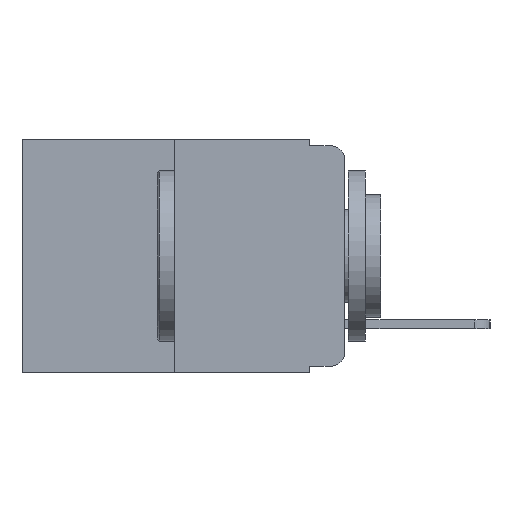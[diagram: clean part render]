
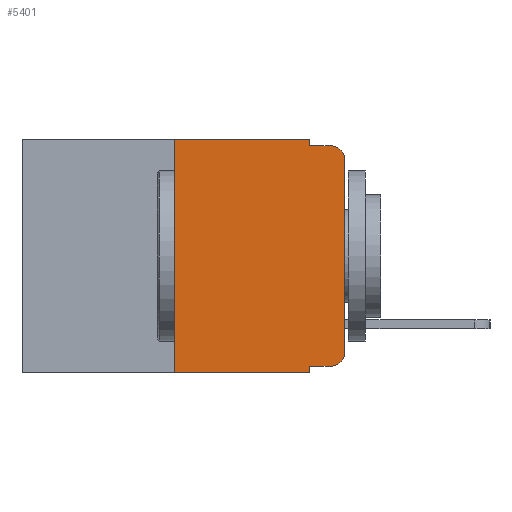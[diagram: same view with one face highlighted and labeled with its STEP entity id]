
A CAD part, left-side view. The second image highlights one B-rep face of the part: STEP entity #5401.
In plain terms, the highlighted planar face has unit normal (-1, 0, 0).
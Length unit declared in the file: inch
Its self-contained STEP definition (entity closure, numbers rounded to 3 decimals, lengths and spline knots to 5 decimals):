
#110 = VERTEX_POINT ( 'NONE', #2199 ) ;
#299 = DIRECTION ( 'NONE',  ( 0., 0., 1. ) ) ;
#365 = CARTESIAN_POINT ( 'NONE',  ( 0., 0.02, -0.01 ) ) ;
#613 = EDGE_CURVE ( 'NONE', #12020, #21949, #14878, .T. ) ;
#1210 = AXIS2_PLACEMENT_3D ( 'NONE', #22900, #11260, #24784 ) ;
#1240 = AXIS2_PLACEMENT_3D ( 'NONE', #11930, #15822, #15746 ) ;
#1742 = CARTESIAN_POINT ( 'NONE',  ( 0., 0.051, -0.01 ) ) ;
#2199 = CARTESIAN_POINT ( 'NONE',  ( 0., 0., -0.03 ) ) ;
#2797 = CARTESIAN_POINT ( 'NONE',  ( 0., 0.051, -0.333 ) ) ;
#2914 = VECTOR ( 'NONE', #299, 39.37008 ) ;
#2968 = DIRECTION ( 'NONE',  ( 0., 0., -1. ) ) ;
#3249 = VECTOR ( 'NONE', #24885, 39.37008 ) ;
#3741 = ORIENTED_EDGE ( 'NONE', *, *, #14303, .F. ) ;
#3817 = ORIENTED_EDGE ( 'NONE', *, *, #24107, .T. ) ;
#4139 = VECTOR ( 'NONE', #13583, 39.37008 ) ;
#5282 = CARTESIAN_POINT ( 'NONE',  ( 0., 0.051, -0.343 ) ) ;
#5379 = VECTOR ( 'NONE', #2968, 39.37008 ) ;
#5401 = ADVANCED_FACE ( 'NONE', ( #16788 ), #16209, .F. ) ;
#5691 = EDGE_CURVE ( 'NONE', #10953, #9320, #20780, .T. ) ;
#5709 = CARTESIAN_POINT ( 'NONE',  ( 0., 0.02, -0.313 ) ) ;
#6257 = CARTESIAN_POINT ( 'NONE',  ( 0., 0.051, 0. ) ) ;
#6479 = VERTEX_POINT ( 'NONE', #365 ) ;
#6507 = VERTEX_POINT ( 'NONE', #17838 ) ;
#7349 = VERTEX_POINT ( 'NONE', #8940 ) ;
#7655 = DIRECTION ( 'NONE',  ( 0., 0., -1. ) ) ;
#8054 = CARTESIAN_POINT ( 'NONE',  ( 0., 0., 0. ) ) ;
#8216 = LINE ( 'NONE', #22053, #17794 ) ;
#8354 = LINE ( 'NONE', #1742, #3249 ) ;
#8837 = CARTESIAN_POINT ( 'NONE',  ( 0., 0.051, -0.333 ) ) ;
#8940 = CARTESIAN_POINT ( 'NONE',  ( 0., 0.25, -0.343 ) ) ;
#8973 = EDGE_CURVE ( 'NONE', #10953, #19774, #20629, .T. ) ;
#9078 = VERTEX_POINT ( 'NONE', #19848 ) ;
#9320 = VERTEX_POINT ( 'NONE', #5282 ) ;
#10343 = VECTOR ( 'NONE', #18164, 39.37008 ) ;
#10953 = VERTEX_POINT ( 'NONE', #8837 ) ;
#11128 = ORIENTED_EDGE ( 'NONE', *, *, #24139, .T. ) ;
#11260 = DIRECTION ( 'NONE',  ( -1., 0., 0. ) ) ;
#11719 = CARTESIAN_POINT ( 'NONE',  ( 0., 0.473, -0.343 ) ) ;
#11804 = EDGE_CURVE ( 'NONE', #9078, #6479, #8354, .T. ) ;
#11930 = CARTESIAN_POINT ( 'NONE',  ( 0., 0.473, 0. ) ) ;
#12020 = VERTEX_POINT ( 'NONE', #16234 ) ;
#12696 = EDGE_CURVE ( 'NONE', #110, #6479, #20682, .T. ) ;
#12757 = CIRCLE ( 'NONE', #14114, 0.02 ) ;
#13583 = DIRECTION ( 'NONE',  ( 0., -1., 0. ) ) ;
#13606 = VECTOR ( 'NONE', #16019, 39.37008 ) ;
#14099 = CARTESIAN_POINT ( 'NONE',  ( 0., 0.25, 0. ) ) ;
#14114 = AXIS2_PLACEMENT_3D ( 'NONE', #5709, #19171, #7655 ) ;
#14237 = LINE ( 'NONE', #11719, #4139 ) ;
#14303 = EDGE_CURVE ( 'NONE', #21949, #9078, #8216, .T. ) ;
#14865 = ORIENTED_EDGE ( 'NONE', *, *, #8973, .T. ) ;
#14878 = LINE ( 'NONE', #24428, #24662 ) ;
#15746 = DIRECTION ( 'NONE',  ( 0., 0., -1. ) ) ;
#15822 = DIRECTION ( 'NONE',  ( 1., 0., 0. ) ) ;
#16019 = DIRECTION ( 'NONE',  ( 0., 0., 1. ) ) ;
#16209 = PLANE ( 'NONE',  #1240 ) ;
#16234 = CARTESIAN_POINT ( 'NONE',  ( 0., 0.25, 0. ) ) ;
#16788 = FACE_OUTER_BOUND ( 'NONE', #18303, .T. ) ;
#17525 = ORIENTED_EDGE ( 'NONE', *, *, #613, .F. ) ;
#17794 = VECTOR ( 'NONE', #23969, 39.37008 ) ;
#17838 = CARTESIAN_POINT ( 'NONE',  ( 0., 0., -0.313 ) ) ;
#18164 = DIRECTION ( 'NONE',  ( 0., -1., 0. ) ) ;
#18247 = ORIENTED_EDGE ( 'NONE', *, *, #5691, .F. ) ;
#18300 = ORIENTED_EDGE ( 'NONE', *, *, #23982, .T. ) ;
#18303 = EDGE_LOOP ( 'NONE', ( #11128, #20539, #22431, #3741, #17525, #22521, #3817, #18247, #14865, #18300 ) ) ;
#18834 = LINE ( 'NONE', #14099, #13606 ) ;
#18868 = LINE ( 'NONE', #8054, #2914 ) ;
#19171 = DIRECTION ( 'NONE',  ( -1., 0., 0. ) ) ;
#19272 = EDGE_CURVE ( 'NONE', #7349, #12020, #18834, .T. ) ;
#19774 = VERTEX_POINT ( 'NONE', #23449 ) ;
#19848 = CARTESIAN_POINT ( 'NONE',  ( 0., 0.051, -0.01 ) ) ;
#20539 = ORIENTED_EDGE ( 'NONE', *, *, #12696, .T. ) ;
#20629 = LINE ( 'NONE', #2797, #10343 ) ;
#20682 = CIRCLE ( 'NONE', #1210, 0.02 ) ;
#20780 = LINE ( 'NONE', #6257, #5379 ) ;
#21949 = VERTEX_POINT ( 'NONE', #24093 ) ;
#22053 = CARTESIAN_POINT ( 'NONE',  ( 0., 0.051, 0. ) ) ;
#22431 = ORIENTED_EDGE ( 'NONE', *, *, #11804, .F. ) ;
#22521 = ORIENTED_EDGE ( 'NONE', *, *, #19272, .F. ) ;
#22900 = CARTESIAN_POINT ( 'NONE',  ( 0., 0.02, -0.03 ) ) ;
#23449 = CARTESIAN_POINT ( 'NONE',  ( 0., 0.02, -0.333 ) ) ;
#23666 = DIRECTION ( 'NONE',  ( 0., -1., 0. ) ) ;
#23969 = DIRECTION ( 'NONE',  ( 0., 0., -1. ) ) ;
#23982 = EDGE_CURVE ( 'NONE', #19774, #6507, #12757, .T. ) ;
#24093 = CARTESIAN_POINT ( 'NONE',  ( 0., 0.051, 0. ) ) ;
#24107 = EDGE_CURVE ( 'NONE', #7349, #9320, #14237, .T. ) ;
#24139 = EDGE_CURVE ( 'NONE', #6507, #110, #18868, .T. ) ;
#24428 = CARTESIAN_POINT ( 'NONE',  ( 0., 0.473, 0. ) ) ;
#24662 = VECTOR ( 'NONE', #23666, 39.37008 ) ;
#24784 = DIRECTION ( 'NONE',  ( 0., 0., -1. ) ) ;
#24885 = DIRECTION ( 'NONE',  ( 0., -1., 0. ) ) ;
